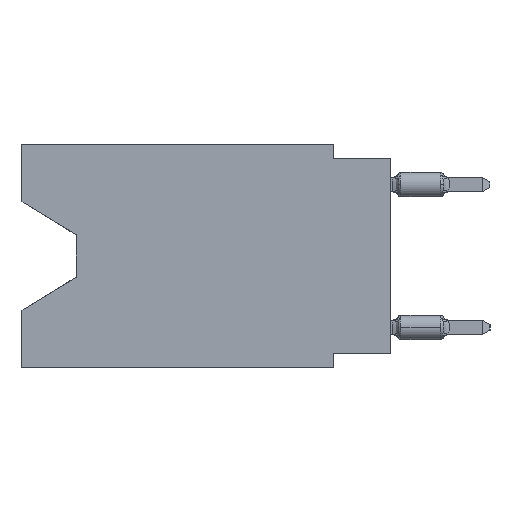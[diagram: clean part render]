
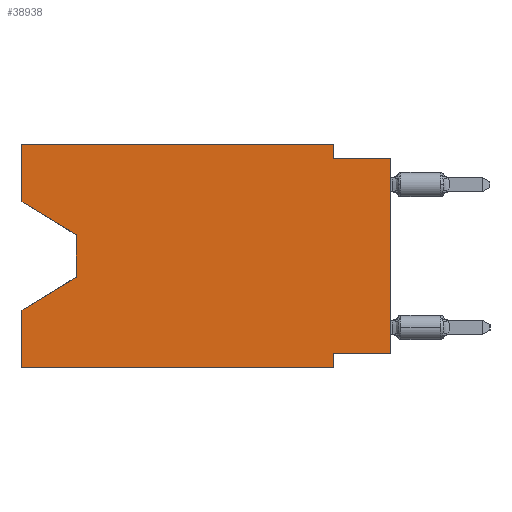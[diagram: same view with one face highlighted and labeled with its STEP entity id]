
A CAD part, left-side view. The second image highlights one B-rep face of the part: STEP entity #38938.
In plain terms, the highlighted planar face has unit normal (-1, 0, 0).
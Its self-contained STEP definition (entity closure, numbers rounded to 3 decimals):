
#671 = CARTESIAN_POINT ( 'NONE',  ( 0., 0., -9.271 ) ) ;
#1276 = PLANE ( 'NONE',  #18381 ) ;
#1308 = DIRECTION ( 'NONE',  ( 0., 0., -1. ) ) ;
#1442 = ORIENTED_EDGE ( 'NONE', *, *, #32734, .T. ) ;
#1604 = DIRECTION ( 'NONE',  ( 0., 0., 1. ) ) ;
#2535 = CARTESIAN_POINT ( 'NONE',  ( 0., 16.383, -2.546 ) ) ;
#3669 = EDGE_CURVE ( 'NONE', #42184, #51566, #63572, .T. ) ;
#3899 = ORIENTED_EDGE ( 'NONE', *, *, #8497, .T. ) ;
#4959 = LINE ( 'NONE', #42548, #63596 ) ;
#5389 = DIRECTION ( 'NONE',  ( 0., 0.855, -0.519 ) ) ;
#6718 = LINE ( 'NONE', #27577, #54692 ) ;
#7000 = VERTEX_POINT ( 'NONE', #10434 ) ;
#7743 = DIRECTION ( 'NONE',  ( 0., 0., -1. ) ) ;
#7821 = CARTESIAN_POINT ( 'NONE',  ( 0., 16.383, 0. ) ) ;
#8058 = ORIENTED_EDGE ( 'NONE', *, *, #66547, .T. ) ;
#8497 = EDGE_CURVE ( 'NONE', #64677, #7000, #53973, .T. ) ;
#9650 = VERTEX_POINT ( 'NONE', #33083 ) ;
#10434 = CARTESIAN_POINT ( 'NONE',  ( 0., 0., -0.635 ) ) ;
#10535 = CARTESIAN_POINT ( 'NONE',  ( 0., 16.383, 0. ) ) ;
#11592 = LINE ( 'NONE', #7821, #43483 ) ;
#12460 = EDGE_CURVE ( 'NONE', #42184, #15438, #37807, .T. ) ;
#15438 = VERTEX_POINT ( 'NONE', #60429 ) ;
#17326 = LINE ( 'NONE', #59072, #62094 ) ;
#17794 = EDGE_CURVE ( 'NONE', #34290, #46509, #54535, .T. ) ;
#18381 = AXIS2_PLACEMENT_3D ( 'NONE', #38844, #53609, #43310 ) ;
#19628 = ORIENTED_EDGE ( 'NONE', *, *, #32622, .F. ) ;
#20066 = ORIENTED_EDGE ( 'NONE', *, *, #17794, .T. ) ;
#20268 = LINE ( 'NONE', #41126, #37477 ) ;
#20914 = ORIENTED_EDGE ( 'NONE', *, *, #55974, .F. ) ;
#25521 = ORIENTED_EDGE ( 'NONE', *, *, #40030, .F. ) ;
#27577 = CARTESIAN_POINT ( 'NONE',  ( 0., 16.383, 0. ) ) ;
#28900 = CARTESIAN_POINT ( 'NONE',  ( 0., 16.383, -9.906 ) ) ;
#29469 = DIRECTION ( 'NONE',  ( 0., -1., 0. ) ) ;
#30074 = ORIENTED_EDGE ( 'NONE', *, *, #60920, .F. ) ;
#31460 = VECTOR ( 'NONE', #29469, 1000. ) ;
#31878 = DIRECTION ( 'NONE',  ( 0., 1., 0. ) ) ;
#32024 = VERTEX_POINT ( 'NONE', #49088 ) ;
#32622 = EDGE_CURVE ( 'NONE', #9650, #7000, #65089, .T. ) ;
#32719 = FACE_OUTER_BOUND ( 'NONE', #61726, .T. ) ;
#32734 = EDGE_CURVE ( 'NONE', #46509, #51284, #56500, .T. ) ;
#33058 = CARTESIAN_POINT ( 'NONE',  ( 0., 16.383, 0. ) ) ;
#33083 = CARTESIAN_POINT ( 'NONE',  ( 0., 2.54, -0.635 ) ) ;
#33153 = CARTESIAN_POINT ( 'NONE',  ( 0., 13.97, -5.893 ) ) ;
#34290 = VERTEX_POINT ( 'NONE', #44505 ) ;
#35597 = CARTESIAN_POINT ( 'NONE',  ( 0., 13.97, -4.013 ) ) ;
#37477 = VECTOR ( 'NONE', #31878, 1000. ) ;
#37807 = LINE ( 'NONE', #28900, #50270 ) ;
#38043 = CARTESIAN_POINT ( 'NONE',  ( 0., 13.97, -4.013 ) ) ;
#38534 = CARTESIAN_POINT ( 'NONE',  ( 0., 2.54, 0. ) ) ;
#38582 = EDGE_CURVE ( 'NONE', #60245, #32024, #11592, .T. ) ;
#38844 = CARTESIAN_POINT ( 'NONE',  ( 0., 16.383, 0. ) ) ;
#38938 = ADVANCED_FACE ( 'NONE', ( #32719 ), #1276, .F. ) ;
#39360 = CARTESIAN_POINT ( 'NONE',  ( 0., 2.54, -9.271 ) ) ;
#40030 = EDGE_CURVE ( 'NONE', #32024, #9650, #43674, .T. ) ;
#41126 = CARTESIAN_POINT ( 'NONE',  ( 0., 0., -9.271 ) ) ;
#42184 = VERTEX_POINT ( 'NONE', #63159 ) ;
#42548 = CARTESIAN_POINT ( 'NONE',  ( 0., 2.54, -9.906 ) ) ;
#43310 = DIRECTION ( 'NONE',  ( 0., 0., -1. ) ) ;
#43483 = VECTOR ( 'NONE', #63963, 1000. ) ;
#43674 = LINE ( 'NONE', #38534, #52515 ) ;
#44251 = DIRECTION ( 'NONE',  ( 0., -0.855, -0.519 ) ) ;
#44505 = CARTESIAN_POINT ( 'NONE',  ( 0., 16.383, -2.546 ) ) ;
#44641 = DIRECTION ( 'NONE',  ( 0., -1., 0. ) ) ;
#45401 = ORIENTED_EDGE ( 'NONE', *, *, #59174, .F. ) ;
#46313 = ORIENTED_EDGE ( 'NONE', *, *, #38582, .F. ) ;
#46454 = CARTESIAN_POINT ( 'NONE',  ( 0., 16.383, -7.36 ) ) ;
#46509 = VERTEX_POINT ( 'NONE', #38043 ) ;
#46790 = VECTOR ( 'NONE', #47486, 1000. ) ;
#46819 = VECTOR ( 'NONE', #1308, 1000. ) ;
#47337 = VECTOR ( 'NONE', #44251, 1000. ) ;
#47486 = DIRECTION ( 'NONE',  ( 0., 0., 1. ) ) ;
#48505 = DIRECTION ( 'NONE',  ( 0., 0., 1. ) ) ;
#49088 = CARTESIAN_POINT ( 'NONE',  ( 0., 2.54, 0. ) ) ;
#49386 = ORIENTED_EDGE ( 'NONE', *, *, #12460, .T. ) ;
#49512 = CARTESIAN_POINT ( 'NONE',  ( 0., 0., 0. ) ) ;
#50270 = VECTOR ( 'NONE', #44641, 1000. ) ;
#50981 = VERTEX_POINT ( 'NONE', #39360 ) ;
#51284 = VERTEX_POINT ( 'NONE', #33153 ) ;
#51566 = VERTEX_POINT ( 'NONE', #46454 ) ;
#52515 = VECTOR ( 'NONE', #7743, 1000. ) ;
#52692 = VECTOR ( 'NONE', #48505, 1000. ) ;
#53609 = DIRECTION ( 'NONE',  ( 1., 0., 0. ) ) ;
#53973 = LINE ( 'NONE', #49512, #52692 ) ;
#54535 = LINE ( 'NONE', #2535, #47337 ) ;
#54692 = VECTOR ( 'NONE', #1604, 1000. ) ;
#55974 = EDGE_CURVE ( 'NONE', #34290, #60245, #6718, .T. ) ;
#56500 = LINE ( 'NONE', #35597, #46819 ) ;
#59072 = CARTESIAN_POINT ( 'NONE',  ( 0., 13.97, -5.893 ) ) ;
#59174 = EDGE_CURVE ( 'NONE', #50981, #15438, #4959, .T. ) ;
#60245 = VERTEX_POINT ( 'NONE', #33058 ) ;
#60401 = ORIENTED_EDGE ( 'NONE', *, *, #3669, .F. ) ;
#60429 = CARTESIAN_POINT ( 'NONE',  ( 0., 2.54, -9.906 ) ) ;
#60920 = EDGE_CURVE ( 'NONE', #64677, #50981, #20268, .T. ) ;
#60956 = CARTESIAN_POINT ( 'NONE',  ( 0., 0., -0.635 ) ) ;
#61726 = EDGE_LOOP ( 'NONE', ( #20066, #1442, #8058, #60401, #49386, #45401, #30074, #3899, #19628, #25521, #46313, #20914 ) ) ;
#62094 = VECTOR ( 'NONE', #5389, 1000. ) ;
#62098 = DIRECTION ( 'NONE',  ( 0., 0., -1. ) ) ;
#63159 = CARTESIAN_POINT ( 'NONE',  ( 0., 16.383, -9.906 ) ) ;
#63572 = LINE ( 'NONE', #10535, #46790 ) ;
#63596 = VECTOR ( 'NONE', #62098, 1000. ) ;
#63963 = DIRECTION ( 'NONE',  ( 0., -1., 0. ) ) ;
#64677 = VERTEX_POINT ( 'NONE', #671 ) ;
#65089 = LINE ( 'NONE', #60956, #31460 ) ;
#66547 = EDGE_CURVE ( 'NONE', #51284, #51566, #17326, .T. ) ;
